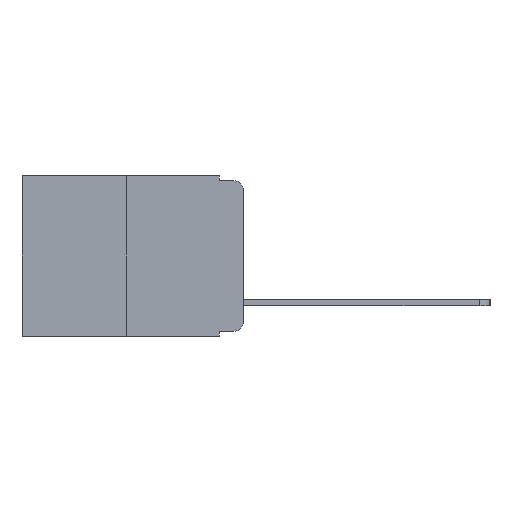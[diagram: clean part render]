
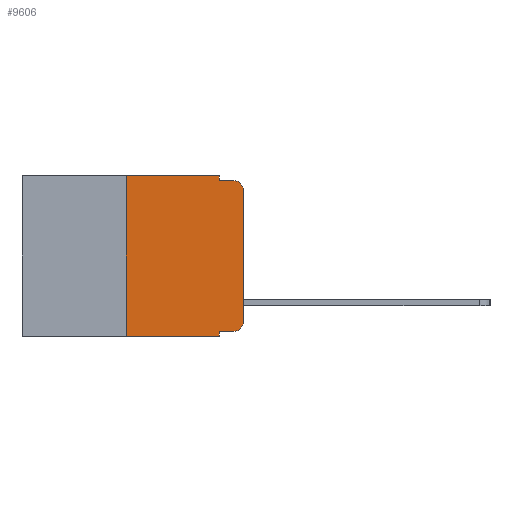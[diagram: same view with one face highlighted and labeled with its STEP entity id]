
A CAD part, left-side view. The second image highlights one B-rep face of the part: STEP entity #9606.
In plain terms, the highlighted planar face has unit normal (-1, 0, 0).
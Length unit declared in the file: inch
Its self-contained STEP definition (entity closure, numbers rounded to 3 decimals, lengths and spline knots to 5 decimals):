
#433 = EDGE_CURVE ( 'NONE', #3245, #6861, #2310, .T. ) ;
#445 = CARTESIAN_POINT ( 'NONE',  ( 0., 0.051, 0. ) ) ;
#512 = AXIS2_PLACEMENT_3D ( 'NONE', #6891, #919, #7857 ) ;
#621 = CARTESIAN_POINT ( 'NONE',  ( 0., 0.02, -0.333 ) ) ;
#758 = ORIENTED_EDGE ( 'NONE', *, *, #3849, .F. ) ;
#797 = VECTOR ( 'NONE', #6783, 39.37008 ) ;
#813 = CARTESIAN_POINT ( 'NONE',  ( 0., 0.473, -0.343 ) ) ;
#919 = DIRECTION ( 'NONE',  ( -1., 0., 0. ) ) ;
#1075 = ORIENTED_EDGE ( 'NONE', *, *, #3157, .F. ) ;
#1111 = EDGE_CURVE ( 'NONE', #7365, #3245, #8005, .T. ) ;
#1332 = CARTESIAN_POINT ( 'NONE',  ( 0., 0.02, -0.313 ) ) ;
#1495 = VERTEX_POINT ( 'NONE', #3147 ) ;
#1538 = LINE ( 'NONE', #1871, #6844 ) ;
#1781 = EDGE_CURVE ( 'NONE', #7365, #7123, #10342, .T. ) ;
#1871 = CARTESIAN_POINT ( 'NONE',  ( 0., 0., 0. ) ) ;
#2310 = CIRCLE ( 'NONE', #7965, 0.02 ) ;
#2342 = ORIENTED_EDGE ( 'NONE', *, *, #433, .T. ) ;
#2361 = DIRECTION ( 'NONE',  ( 0., 0., -1. ) ) ;
#2461 = EDGE_CURVE ( 'NONE', #7661, #1495, #3386, .T. ) ;
#2493 = VERTEX_POINT ( 'NONE', #8470 ) ;
#2760 = CARTESIAN_POINT ( 'NONE',  ( 0., 0.051, -0.01 ) ) ;
#2841 = EDGE_LOOP ( 'NONE', ( #8048, #5785, #758, #1075, #3794, #9534, #11991, #7301, #9823, #2342 ) ) ;
#2869 = DIRECTION ( 'NONE',  ( 0., 0., 1. ) ) ;
#2896 = PLANE ( 'NONE',  #3707 ) ;
#3147 = CARTESIAN_POINT ( 'NONE',  ( 0., 0.25, 0. ) ) ;
#3157 = EDGE_CURVE ( 'NONE', #2493, #5251, #12472, .T. ) ;
#3245 = VERTEX_POINT ( 'NONE', #621 ) ;
#3386 = LINE ( 'NONE', #4528, #10755 ) ;
#3558 = DIRECTION ( 'NONE',  ( 0., -1., 0. ) ) ;
#3707 = AXIS2_PLACEMENT_3D ( 'NONE', #11516, #9697, #3927 ) ;
#3794 = ORIENTED_EDGE ( 'NONE', *, *, #5664, .F. ) ;
#3849 = EDGE_CURVE ( 'NONE', #5251, #11013, #8226, .T. ) ;
#3927 = DIRECTION ( 'NONE',  ( 0., 0., -1. ) ) ;
#4494 = EDGE_CURVE ( 'NONE', #9318, #11013, #11434, .T. ) ;
#4528 = CARTESIAN_POINT ( 'NONE',  ( 0., 0.25, 0. ) ) ;
#4631 = FACE_OUTER_BOUND ( 'NONE', #2841, .T. ) ;
#4697 = CARTESIAN_POINT ( 'NONE',  ( 0., 0.473, 0. ) ) ;
#4920 = VECTOR ( 'NONE', #6440, 39.37008 ) ;
#5157 = EDGE_CURVE ( 'NONE', #6861, #9318, #1538, .T. ) ;
#5251 = VERTEX_POINT ( 'NONE', #7931 ) ;
#5257 = VECTOR ( 'NONE', #5521, 39.37008 ) ;
#5354 = VECTOR ( 'NONE', #9571, 39.37008 ) ;
#5521 = DIRECTION ( 'NONE',  ( 0., 0., -1. ) ) ;
#5664 = EDGE_CURVE ( 'NONE', #1495, #2493, #9088, .T. ) ;
#5785 = ORIENTED_EDGE ( 'NONE', *, *, #4494, .T. ) ;
#6440 = DIRECTION ( 'NONE',  ( 0., 0., -1. ) ) ;
#6532 = VECTOR ( 'NONE', #7621, 39.37008 ) ;
#6783 = DIRECTION ( 'NONE',  ( 0., -1., 0. ) ) ;
#6844 = VECTOR ( 'NONE', #2869, 39.37008 ) ;
#6861 = VERTEX_POINT ( 'NONE', #8991 ) ;
#6891 = CARTESIAN_POINT ( 'NONE',  ( 0., 0.02, -0.03 ) ) ;
#7123 = VERTEX_POINT ( 'NONE', #8406 ) ;
#7301 = ORIENTED_EDGE ( 'NONE', *, *, #1781, .F. ) ;
#7365 = VERTEX_POINT ( 'NONE', #8736 ) ;
#7434 = CARTESIAN_POINT ( 'NONE',  ( 0., 0.25, -0.343 ) ) ;
#7621 = DIRECTION ( 'NONE',  ( 0., -1., 0. ) ) ;
#7661 = VERTEX_POINT ( 'NONE', #7434 ) ;
#7701 = VECTOR ( 'NONE', #3558, 39.37008 ) ;
#7857 = DIRECTION ( 'NONE',  ( 0., 0., -1. ) ) ;
#7931 = CARTESIAN_POINT ( 'NONE',  ( 0., 0.051, -0.01 ) ) ;
#7965 = AXIS2_PLACEMENT_3D ( 'NONE', #1332, #8261, #2361 ) ;
#8005 = LINE ( 'NONE', #10299, #7701 ) ;
#8048 = ORIENTED_EDGE ( 'NONE', *, *, #5157, .T. ) ;
#8226 = LINE ( 'NONE', #2760, #5354 ) ;
#8261 = DIRECTION ( 'NONE',  ( -1., 0., 0. ) ) ;
#8406 = CARTESIAN_POINT ( 'NONE',  ( 0., 0.051, -0.343 ) ) ;
#8470 = CARTESIAN_POINT ( 'NONE',  ( 0., 0.051, 0. ) ) ;
#8686 = LINE ( 'NONE', #813, #797 ) ;
#8736 = CARTESIAN_POINT ( 'NONE',  ( 0., 0.051, -0.333 ) ) ;
#8991 = CARTESIAN_POINT ( 'NONE',  ( 0., 0., -0.313 ) ) ;
#9088 = LINE ( 'NONE', #4697, #6532 ) ;
#9318 = VERTEX_POINT ( 'NONE', #12042 ) ;
#9534 = ORIENTED_EDGE ( 'NONE', *, *, #2461, .F. ) ;
#9571 = DIRECTION ( 'NONE',  ( 0., -1., 0. ) ) ;
#9606 = ADVANCED_FACE ( 'NONE', ( #4631 ), #2896, .F. ) ;
#9697 = DIRECTION ( 'NONE',  ( 1., 0., 0. ) ) ;
#9823 = ORIENTED_EDGE ( 'NONE', *, *, #1111, .T. ) ;
#9932 = CARTESIAN_POINT ( 'NONE',  ( 0., 0.02, -0.01 ) ) ;
#10299 = CARTESIAN_POINT ( 'NONE',  ( 0., 0.051, -0.333 ) ) ;
#10342 = LINE ( 'NONE', #12133, #5257 ) ;
#10755 = VECTOR ( 'NONE', #12124, 39.37008 ) ;
#10823 = EDGE_CURVE ( 'NONE', #7661, #7123, #8686, .T. ) ;
#11013 = VERTEX_POINT ( 'NONE', #9932 ) ;
#11434 = CIRCLE ( 'NONE', #512, 0.02 ) ;
#11516 = CARTESIAN_POINT ( 'NONE',  ( 0., 0.473, 0. ) ) ;
#11991 = ORIENTED_EDGE ( 'NONE', *, *, #10823, .T. ) ;
#12042 = CARTESIAN_POINT ( 'NONE',  ( 0., 0., -0.03 ) ) ;
#12124 = DIRECTION ( 'NONE',  ( 0., 0., 1. ) ) ;
#12133 = CARTESIAN_POINT ( 'NONE',  ( 0., 0.051, 0. ) ) ;
#12472 = LINE ( 'NONE', #445, #4920 ) ;
